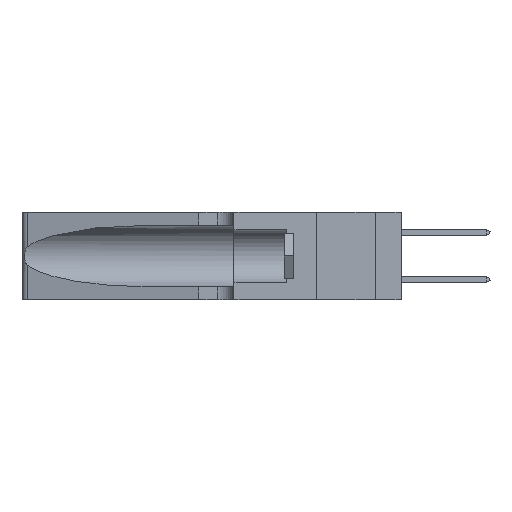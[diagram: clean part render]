
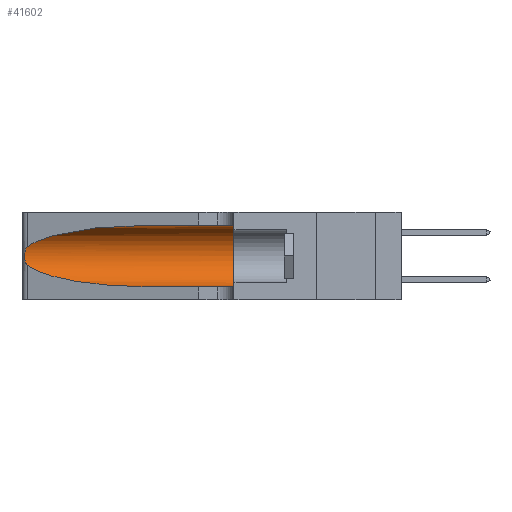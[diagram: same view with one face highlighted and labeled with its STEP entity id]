
A CAD part, left-side view. The second image highlights one B-rep face of the part: STEP entity #41602.
In plain terms, the highlighted cylindrical face has radius 3.308 mm (diameter 6.617 mm), a partial arc.
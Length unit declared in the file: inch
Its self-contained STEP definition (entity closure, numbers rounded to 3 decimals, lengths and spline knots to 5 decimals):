
#1460 = CIRCLE ( 'NONE', #6520, 0.13025 ) ;
#1895 = ORIENTED_EDGE ( 'NONE', *, *, #5439, .F. ) ;
#2884 = CARTESIAN_POINT ( 'NONE',  ( 0.25639, 1.23184, 0.21858 ) ) ;
#3040 = CARTESIAN_POINT ( 'NONE',  ( 0.25487, 1.22718, 0.14631 ) ) ;
#3644 = VERTEX_POINT ( 'NONE', #32200 ) ;
#4199 = DIRECTION ( 'NONE',  ( 0., -1., 0. ) ) ;
#4222 = DIRECTION ( 'NONE',  ( 0., 1., 0. ) ) ;
#4263 = CARTESIAN_POINT ( 'NONE',  ( 0.1305, 1.61858, 0.31525 ) ) ;
#5439 = EDGE_CURVE ( 'NONE', #20213, #9003, #1460, .T. ) ;
#6520 = AXIS2_PLACEMENT_3D ( 'NONE', #26296, #4222, #29969 ) ;
#7963 = DIRECTION ( 'NONE',  ( 0., 0., -1. ) ) ;
#8373 = ORIENTED_EDGE ( 'NONE', *, *, #24268, .T. ) ;
#9003 = VERTEX_POINT ( 'NONE', #30060 ) ;
#9297 = CARTESIAN_POINT ( 'NONE',  ( 0.2373, 1.15595, 0.08982 ) ) ;
#10273 = B_SPLINE_CURVE_WITH_KNOTS ( 'NONE', 3,
 ( #32144, #28636, #2884, #32298, #10304, #36004, #13992, #39699, #17706, #43398, #21376, #47091, #25082, #3040 ),
 .UNSPECIFIED., .F., .F.,
 ( 4, 2, 2, 2, 2, 2, 4 ),
 ( 0., 0.00027, 0.00053, 0.00107, 0.0016, 0.00187, 0.00214 ),
 .UNSPECIFIED. ) ;
#10304 = CARTESIAN_POINT ( 'NONE',  ( 0.25854, 1.2359, 0.20912 ) ) ;
#10779 = CARTESIAN_POINT ( 'NONE',  ( 0.25487, 1.22718, 0.22369 ) ) ;
#12524 = AXIS2_PLACEMENT_3D ( 'NONE', #33505, #29989, #7963 ) ;
#13992 = CARTESIAN_POINT ( 'NONE',  ( 0.26075, 1.23896, 0.19203 ) ) ;
#15668 = VECTOR ( 'NONE', #26329, 39.37008 ) ;
#16700 = CARTESIAN_POINT ( 'NONE',  ( 0.18966, 0.96281, 0.05475 ) ) ;
#17706 = CARTESIAN_POINT ( 'NONE',  ( 0.26017, 1.23833, 0.17102 ) ) ;
#18870 = LINE ( 'NONE', #33613, #37255 ) ;
#20213 = VERTEX_POINT ( 'NONE', #46665 ) ;
#21376 = CARTESIAN_POINT ( 'NONE',  ( 0.25789, 1.23486, 0.15765 ) ) ;
#22503 = EDGE_CURVE ( 'NONE', #47387, #9003, #18870, .T. ) ;
#23834 =( BOUNDED_CURVE ( )  B_SPLINE_CURVE ( 3, ( #29124, #47429, #32796, #10779 ),
 .UNSPECIFIED., .F., .F. ) 
 B_SPLINE_CURVE_WITH_KNOTS ( ( 4, 4 ),
 ( 1.5708, 2.84003 ),
 .UNSPECIFIED. ) 
 CURVE ( )  GEOMETRIC_REPRESENTATION_ITEM ( )  RATIONAL_B_SPLINE_CURVE ( ( 1., 0.87, 0.87, 1. ) ) 
 REPRESENTATION_ITEM ( '' )  );
#23923 = FACE_OUTER_BOUND ( 'NONE', #34844, .T. ) ;
#24268 = EDGE_CURVE ( 'NONE', #28180, #29841, #10273, .T. ) ;
#24749 = EDGE_CURVE ( 'NONE', #29841, #47387, #40885, .T. ) ;
#25082 = CARTESIAN_POINT ( 'NONE',  ( 0.25555, 1.22993, 0.14849 ) ) ;
#26296 = CARTESIAN_POINT ( 'NONE',  ( 0.1305, 0.35, 0.185 ) ) ;
#26329 = DIRECTION ( 'NONE',  ( 0., -1., 0. ) ) ;
#26614 = LINE ( 'NONE', #4263, #15668 ) ;
#27646 = CARTESIAN_POINT ( 'NONE',  ( 0.25487, 1.22718, 0.14631 ) ) ;
#27918 = EDGE_CURVE ( 'NONE', #3644, #28180, #23834, .T. ) ;
#28180 = VERTEX_POINT ( 'NONE', #41621 ) ;
#28614 = ORIENTED_EDGE ( 'NONE', *, *, #27918, .T. ) ;
#28636 = CARTESIAN_POINT ( 'NONE',  ( 0.25555, 1.22994, 0.2215 ) ) ;
#29124 = CARTESIAN_POINT ( 'NONE',  ( 0.1305, 0.72297, 0.31525 ) ) ;
#29841 = VERTEX_POINT ( 'NONE', #32147 ) ;
#29969 = DIRECTION ( 'NONE',  ( 0., 0., 1. ) ) ;
#29989 = DIRECTION ( 'NONE',  ( 0., -1., 0. ) ) ;
#30060 = CARTESIAN_POINT ( 'NONE',  ( 0.1305, 0.35, 0.05475 ) ) ;
#30519 = CARTESIAN_POINT ( 'NONE',  ( 0.1305, 0.72297, 0.05475 ) ) ;
#31377 = CYLINDRICAL_SURFACE ( 'NONE', #12524, 0.13025 ) ;
#32144 = CARTESIAN_POINT ( 'NONE',  ( 0.25487, 1.22718, 0.22369 ) ) ;
#32147 = CARTESIAN_POINT ( 'NONE',  ( 0.25487, 1.22718, 0.14631 ) ) ;
#32200 = CARTESIAN_POINT ( 'NONE',  ( 0.1305, 0.72297, 0.31525 ) ) ;
#32298 = CARTESIAN_POINT ( 'NONE',  ( 0.25787, 1.23484, 0.2124 ) ) ;
#32796 = CARTESIAN_POINT ( 'NONE',  ( 0.2373, 1.15595, 0.28018 ) ) ;
#33505 = CARTESIAN_POINT ( 'NONE',  ( 0.1305, 1.61858, 0.185 ) ) ;
#33613 = CARTESIAN_POINT ( 'NONE',  ( 0.1305, 1.61858, 0.05475 ) ) ;
#34844 = EDGE_LOOP ( 'NONE', ( #28614, #8373, #39064, #44837, #1895, #36833 ) ) ;
#36004 = CARTESIAN_POINT ( 'NONE',  ( 0.26018, 1.23835, 0.19895 ) ) ;
#36833 = ORIENTED_EDGE ( 'NONE', *, *, #43558, .F. ) ;
#37255 = VECTOR ( 'NONE', #4199, 39.37008 ) ;
#39064 = ORIENTED_EDGE ( 'NONE', *, *, #24749, .T. ) ;
#39699 = CARTESIAN_POINT ( 'NONE',  ( 0.26075, 1.23896, 0.178 ) ) ;
#40885 =( BOUNDED_CURVE ( )  B_SPLINE_CURVE ( 3, ( #27646, #9297, #16700, #42407 ),
 .UNSPECIFIED., .F., .T. ) 
 B_SPLINE_CURVE_WITH_KNOTS ( ( 4, 4 ),
 ( 3.44316, 4.71239 ),
 .UNSPECIFIED. ) 
 CURVE ( )  GEOMETRIC_REPRESENTATION_ITEM ( )  RATIONAL_B_SPLINE_CURVE ( ( 1., 0.87, 0.87, 1. ) ) 
 REPRESENTATION_ITEM ( '' )  );
#41602 = ADVANCED_FACE ( 'NONE', ( #23923 ), #31377, .F. ) ;
#41621 = CARTESIAN_POINT ( 'NONE',  ( 0.25487, 1.22718, 0.22369 ) ) ;
#42407 = CARTESIAN_POINT ( 'NONE',  ( 0.1305, 0.72297, 0.05475 ) ) ;
#43398 = CARTESIAN_POINT ( 'NONE',  ( 0.25856, 1.23593, 0.16098 ) ) ;
#43558 = EDGE_CURVE ( 'NONE', #3644, #20213, #26614, .T. ) ;
#44837 = ORIENTED_EDGE ( 'NONE', *, *, #22503, .T. ) ;
#46665 = CARTESIAN_POINT ( 'NONE',  ( 0.1305, 0.35, 0.31525 ) ) ;
#47091 = CARTESIAN_POINT ( 'NONE',  ( 0.25639, 1.23186, 0.15144 ) ) ;
#47387 = VERTEX_POINT ( 'NONE', #30519 ) ;
#47429 = CARTESIAN_POINT ( 'NONE',  ( 0.18966, 0.96281, 0.31525 ) ) ;
